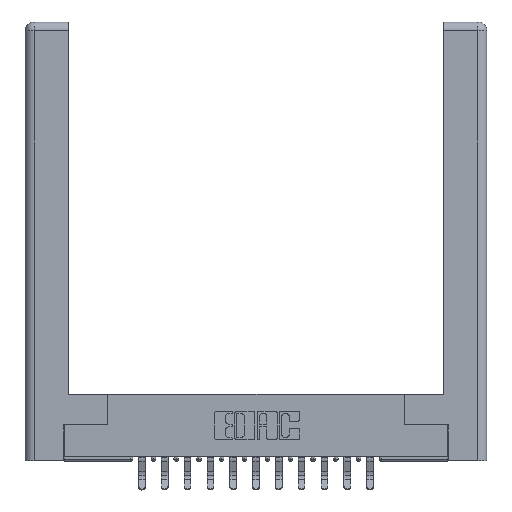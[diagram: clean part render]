
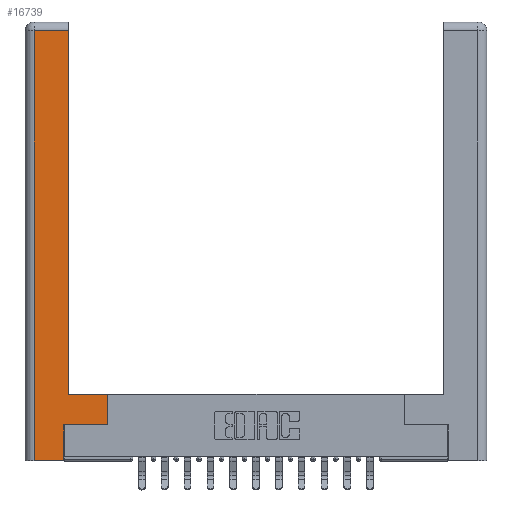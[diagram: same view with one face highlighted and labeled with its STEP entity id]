
A CAD part, top view. The second image highlights one B-rep face of the part: STEP entity #16739.
In plain terms, the highlighted planar face has unit normal (0, 0, 1).
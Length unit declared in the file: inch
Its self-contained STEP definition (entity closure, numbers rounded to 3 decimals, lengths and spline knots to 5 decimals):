
#526 = ORIENTED_EDGE ( 'NONE', *, *, #11803, .T. ) ;
#535 = ORIENTED_EDGE ( 'NONE', *, *, #14041, .T. ) ;
#794 = EDGE_CURVE ( 'NONE', #6537, #1636, #13844, .T. ) ;
#1112 = DIRECTION ( 'NONE',  ( 0., 1., 0. ) ) ;
#1124 = DIRECTION ( 'NONE',  ( 1., 0., 0. ) ) ;
#1521 = DIRECTION ( 'NONE',  ( -1., 0., 0. ) ) ;
#1636 = VERTEX_POINT ( 'NONE', #17983 ) ;
#2555 = CARTESIAN_POINT ( 'NONE',  ( 0.0615, 2.94, 0. ) ) ;
#3170 = DIRECTION ( 'NONE',  ( 0., 0., -1. ) ) ;
#3706 = CARTESIAN_POINT ( 'NONE',  ( 0.295, 2.94, 0. ) ) ;
#3757 = CARTESIAN_POINT ( 'NONE',  ( 0.265, 0., 0. ) ) ;
#3827 = CARTESIAN_POINT ( 'NONE',  ( 0.265, 0.245, 0. ) ) ;
#4052 = VECTOR ( 'NONE', #1521, 39.37008 ) ;
#4289 = CARTESIAN_POINT ( 'NONE',  ( 0.295, 3., 0. ) ) ;
#4898 = VERTEX_POINT ( 'NONE', #12127 ) ;
#5224 = CARTESIAN_POINT ( 'NONE',  ( 0., 0., 0. ) ) ;
#5302 = LINE ( 'NONE', #3757, #6857 ) ;
#5461 = ORIENTED_EDGE ( 'NONE', *, *, #7231, .T. ) ;
#5608 = CARTESIAN_POINT ( 'NONE',  ( 0.0615, 0., 0. ) ) ;
#5790 = LINE ( 'NONE', #3827, #13838 ) ;
#5825 = CARTESIAN_POINT ( 'NONE',  ( 0.295, 0.45, 0. ) ) ;
#6108 = AXIS2_PLACEMENT_3D ( 'NONE', #5224, #3170, #6494 ) ;
#6261 = CARTESIAN_POINT ( 'NONE',  ( 0.565, 0.45, 0. ) ) ;
#6306 = EDGE_CURVE ( 'NONE', #7956, #14640, #14353, .T. ) ;
#6494 = DIRECTION ( 'NONE',  ( -1., 0., 0. ) ) ;
#6537 = VERTEX_POINT ( 'NONE', #3706 ) ;
#6760 = EDGE_CURVE ( 'NONE', #16608, #4898, #5790, .T. ) ;
#6797 = CARTESIAN_POINT ( 'NONE',  ( 0.265, 0., 0. ) ) ;
#6857 = VECTOR ( 'NONE', #1124, 39.37008 ) ;
#6887 = DIRECTION ( 'NONE',  ( 1., 0., 0. ) ) ;
#7231 = EDGE_CURVE ( 'NONE', #1636, #14220, #15889, .T. ) ;
#7488 = CARTESIAN_POINT ( 'NONE',  ( 0.565, 0.45, 0. ) ) ;
#7489 = VECTOR ( 'NONE', #1112, 39.37008 ) ;
#7850 = LINE ( 'NONE', #12903, #4052 ) ;
#7864 = EDGE_CURVE ( 'NONE', #14220, #16608, #5302, .T. ) ;
#7956 = VERTEX_POINT ( 'NONE', #11175 ) ;
#10092 = ORIENTED_EDGE ( 'NONE', *, *, #6760, .T. ) ;
#10375 = CARTESIAN_POINT ( 'NONE',  ( 0.0615, 0., 0. ) ) ;
#11175 = CARTESIAN_POINT ( 'NONE',  ( 0.565, 0.245, 0. ) ) ;
#11195 = ORIENTED_EDGE ( 'NONE', *, *, #6306, .T. ) ;
#11630 = EDGE_LOOP ( 'NONE', ( #15300, #12822, #5461, #15883, #10092, #535, #11195, #526 ) ) ;
#11803 = EDGE_CURVE ( 'NONE', #14640, #16331, #7850, .T. ) ;
#11997 = FACE_OUTER_BOUND ( 'NONE', #11630, .T. ) ;
#12127 = CARTESIAN_POINT ( 'NONE',  ( 0.265, 0.245, 0. ) ) ;
#12457 = VECTOR ( 'NONE', #6887, 39.37008 ) ;
#12822 = ORIENTED_EDGE ( 'NONE', *, *, #794, .T. ) ;
#12903 = CARTESIAN_POINT ( 'NONE',  ( 0.295, 0.45, 0. ) ) ;
#13178 = VECTOR ( 'NONE', #17203, 39.37008 ) ;
#13838 = VECTOR ( 'NONE', #16722, 39.37008 ) ;
#13844 = LINE ( 'NONE', #2555, #17685 ) ;
#14012 = PLANE ( 'NONE',  #6108 ) ;
#14041 = EDGE_CURVE ( 'NONE', #4898, #7956, #16301, .T. ) ;
#14220 = VERTEX_POINT ( 'NONE', #10375 ) ;
#14353 = LINE ( 'NONE', #6261, #17922 ) ;
#14640 = VERTEX_POINT ( 'NONE', #7488 ) ;
#14856 = DIRECTION ( 'NONE',  ( 0., 1., 0. ) ) ;
#15279 = DIRECTION ( 'NONE',  ( -1., 0., 0. ) ) ;
#15300 = ORIENTED_EDGE ( 'NONE', *, *, #18129, .T. ) ;
#15883 = ORIENTED_EDGE ( 'NONE', *, *, #7864, .T. ) ;
#15889 = LINE ( 'NONE', #5608, #13178 ) ;
#16301 = LINE ( 'NONE', #17038, #12457 ) ;
#16331 = VERTEX_POINT ( 'NONE', #5825 ) ;
#16608 = VERTEX_POINT ( 'NONE', #6797 ) ;
#16722 = DIRECTION ( 'NONE',  ( 0., 1., 0. ) ) ;
#16739 = ADVANCED_FACE ( 'NONE', ( #11997 ), #14012, .F. ) ;
#17038 = CARTESIAN_POINT ( 'NONE',  ( 0.565, 0.245, 0. ) ) ;
#17203 = DIRECTION ( 'NONE',  ( 0., -1., 0. ) ) ;
#17359 = LINE ( 'NONE', #4289, #7489 ) ;
#17685 = VECTOR ( 'NONE', #15279, 39.37008 ) ;
#17922 = VECTOR ( 'NONE', #14856, 39.37008 ) ;
#17983 = CARTESIAN_POINT ( 'NONE',  ( 0.0615, 2.94, 0. ) ) ;
#18129 = EDGE_CURVE ( 'NONE', #16331, #6537, #17359, .T. ) ;
